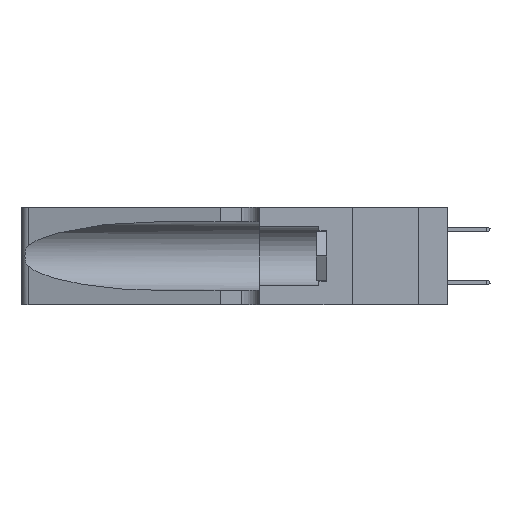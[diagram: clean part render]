
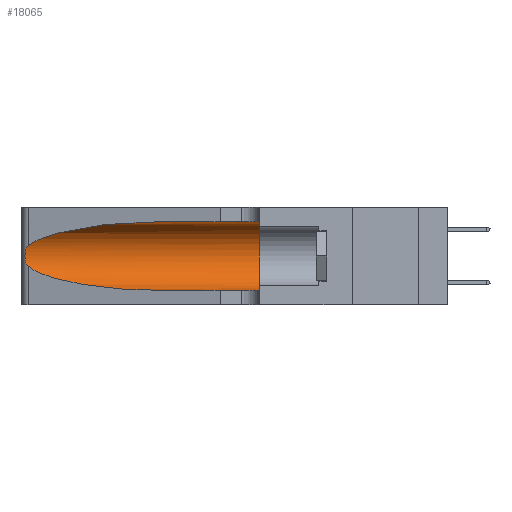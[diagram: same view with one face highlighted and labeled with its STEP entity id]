
A CAD part, left-side view. The second image highlights one B-rep face of the part: STEP entity #18065.
In plain terms, the highlighted cylindrical face has radius 3.308 mm (diameter 6.617 mm), a partial arc.
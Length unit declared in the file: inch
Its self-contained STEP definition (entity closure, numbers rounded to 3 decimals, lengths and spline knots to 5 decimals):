
#172 = CYLINDRICAL_SURFACE ( 'NONE', #28680, 0.13025 ) ;
#810 = CARTESIAN_POINT ( 'NONE',  ( 0.25487, 1.22718, 0.22369 ) ) ;
#1153 = FACE_OUTER_BOUND ( 'NONE', #14754, .T. ) ;
#1333 = CARTESIAN_POINT ( 'NONE',  ( 0.26018, 1.23835, 0.19895 ) ) ;
#2042 = CARTESIAN_POINT ( 'NONE',  ( 0.1305, 0.35, 0.05475 ) ) ;
#2505 = ORIENTED_EDGE ( 'NONE', *, *, #38951, .F. ) ;
#3276 = CIRCLE ( 'NONE', #6187, 0.13025 ) ;
#3531 = CARTESIAN_POINT ( 'NONE',  ( 0.1305, 0.35, 0.185 ) ) ;
#4413 = CARTESIAN_POINT ( 'NONE',  ( 0.26075, 1.23896, 0.178 ) ) ;
#4618 = CARTESIAN_POINT ( 'NONE',  ( 0.1305, 0.72297, 0.05475 ) ) ;
#4902 = ORIENTED_EDGE ( 'NONE', *, *, #29166, .F. ) ;
#6082 = CARTESIAN_POINT ( 'NONE',  ( 0.1305, 1.61858, 0.05475 ) ) ;
#6187 = AXIS2_PLACEMENT_3D ( 'NONE', #3531, #25128, #6649 ) ;
#6359 =( BOUNDED_CURVE ( )  B_SPLINE_CURVE ( 3, ( #38432, #16950, #23096, #4618 ),
 .UNSPECIFIED., .F., .T. ) 
 B_SPLINE_CURVE_WITH_KNOTS ( ( 4, 4 ),
 ( 3.44316, 4.71239 ),
 .UNSPECIFIED. ) 
 CURVE ( )  GEOMETRIC_REPRESENTATION_ITEM ( )  RATIONAL_B_SPLINE_CURVE ( ( 1., 0.87, 0.87, 1. ) ) 
 REPRESENTATION_ITEM ( '' )  );
#6649 = DIRECTION ( 'NONE',  ( 0., 0., 1. ) ) ;
#6908 = CARTESIAN_POINT ( 'NONE',  ( 0.18966, 0.96281, 0.31525 ) ) ;
#7192 = VECTOR ( 'NONE', #23256, 39.37008 ) ;
#7552 = CARTESIAN_POINT ( 'NONE',  ( 0.25856, 1.23593, 0.16098 ) ) ;
#7822 =( BOUNDED_CURVE ( )  B_SPLINE_CURVE ( 3, ( #13120, #6908, #19323, #810 ),
 .UNSPECIFIED., .F., .T. ) 
 B_SPLINE_CURVE_WITH_KNOTS ( ( 4, 4 ),
 ( 1.5708, 2.84003 ),
 .UNSPECIFIED. ) 
 CURVE ( )  GEOMETRIC_REPRESENTATION_ITEM ( )  RATIONAL_B_SPLINE_CURVE ( ( 1., 0.87, 0.87, 1. ) ) 
 REPRESENTATION_ITEM ( '' )  );
#8098 = ORIENTED_EDGE ( 'NONE', *, *, #9304, .T. ) ;
#8523 = ORIENTED_EDGE ( 'NONE', *, *, #10488, .T. ) ;
#9304 = EDGE_CURVE ( 'NONE', #12887, #9495, #32209, .T. ) ;
#9495 = VERTEX_POINT ( 'NONE', #36215 ) ;
#10488 = EDGE_CURVE ( 'NONE', #17435, #12887, #7822, .T. ) ;
#10525 = ORIENTED_EDGE ( 'NONE', *, *, #38538, .T. ) ;
#10658 = CARTESIAN_POINT ( 'NONE',  ( 0.25639, 1.23186, 0.15144 ) ) ;
#10725 = VERTEX_POINT ( 'NONE', #2042 ) ;
#12756 = VERTEX_POINT ( 'NONE', #27336 ) ;
#12887 = VERTEX_POINT ( 'NONE', #21657 ) ;
#13120 = CARTESIAN_POINT ( 'NONE',  ( 0.1305, 0.72297, 0.31525 ) ) ;
#13646 = CARTESIAN_POINT ( 'NONE',  ( 0.25555, 1.22994, 0.2215 ) ) ;
#13783 = CARTESIAN_POINT ( 'NONE',  ( 0.25487, 1.22718, 0.14631 ) ) ;
#14754 = EDGE_LOOP ( 'NONE', ( #8523, #8098, #10525, #37962, #4902, #2505 ) ) ;
#14966 = VERTEX_POINT ( 'NONE', #27499 ) ;
#16735 = CARTESIAN_POINT ( 'NONE',  ( 0.25487, 1.22718, 0.22369 ) ) ;
#16884 = DIRECTION ( 'NONE',  ( 0., 0., -1. ) ) ;
#16950 = CARTESIAN_POINT ( 'NONE',  ( 0.2373, 1.15595, 0.08982 ) ) ;
#17435 = VERTEX_POINT ( 'NONE', #32528 ) ;
#18065 = ADVANCED_FACE ( 'NONE', ( #1153 ), #172, .F. ) ;
#18513 = DIRECTION ( 'NONE',  ( 0., -1., 0. ) ) ;
#19323 = CARTESIAN_POINT ( 'NONE',  ( 0.2373, 1.15595, 0.28018 ) ) ;
#19823 = CARTESIAN_POINT ( 'NONE',  ( 0.25854, 1.2359, 0.20912 ) ) ;
#21657 = CARTESIAN_POINT ( 'NONE',  ( 0.25487, 1.22718, 0.22369 ) ) ;
#22182 = VECTOR ( 'NONE', #18513, 39.37008 ) ;
#22871 = CARTESIAN_POINT ( 'NONE',  ( 0.26075, 1.23896, 0.19203 ) ) ;
#23096 = CARTESIAN_POINT ( 'NONE',  ( 0.18966, 0.96281, 0.05475 ) ) ;
#23256 = DIRECTION ( 'NONE',  ( 0., -1., 0. ) ) ;
#25128 = DIRECTION ( 'NONE',  ( 0., 1., 0. ) ) ;
#25350 = LINE ( 'NONE', #38593, #7192 ) ;
#25990 = CARTESIAN_POINT ( 'NONE',  ( 0.26017, 1.23833, 0.17102 ) ) ;
#27336 = CARTESIAN_POINT ( 'NONE',  ( 0.1305, 0.35, 0.31525 ) ) ;
#27499 = CARTESIAN_POINT ( 'NONE',  ( 0.1305, 0.72297, 0.05475 ) ) ;
#28680 = AXIS2_PLACEMENT_3D ( 'NONE', #32208, #29233, #16884 ) ;
#29087 = CARTESIAN_POINT ( 'NONE',  ( 0.25789, 1.23486, 0.15765 ) ) ;
#29166 = EDGE_CURVE ( 'NONE', #12756, #10725, #3276, .T. ) ;
#29233 = DIRECTION ( 'NONE',  ( 0., -1., 0. ) ) ;
#30190 = EDGE_CURVE ( 'NONE', #14966, #10725, #31337, .T. ) ;
#31337 = LINE ( 'NONE', #6082, #22182 ) ;
#32057 = CARTESIAN_POINT ( 'NONE',  ( 0.25639, 1.23184, 0.21858 ) ) ;
#32193 = CARTESIAN_POINT ( 'NONE',  ( 0.25555, 1.22993, 0.14849 ) ) ;
#32208 = CARTESIAN_POINT ( 'NONE',  ( 0.1305, 1.61858, 0.185 ) ) ;
#32209 = B_SPLINE_CURVE_WITH_KNOTS ( 'NONE', 3,
 ( #16735, #13646, #32057, #38234, #19823, #1333, #22871, #4413, #25990, #7552, #29087, #10658, #32193, #13783 ),
 .UNSPECIFIED., .F., .F.,
 ( 4, 2, 2, 2, 2, 2, 4 ),
 ( 0., 0.00027, 0.00053, 0.00107, 0.0016, 0.00187, 0.00214 ),
 .UNSPECIFIED. ) ;
#32528 = CARTESIAN_POINT ( 'NONE',  ( 0.1305, 0.72297, 0.31525 ) ) ;
#36215 = CARTESIAN_POINT ( 'NONE',  ( 0.25487, 1.22718, 0.14631 ) ) ;
#37962 = ORIENTED_EDGE ( 'NONE', *, *, #30190, .T. ) ;
#38234 = CARTESIAN_POINT ( 'NONE',  ( 0.25787, 1.23484, 0.2124 ) ) ;
#38432 = CARTESIAN_POINT ( 'NONE',  ( 0.25487, 1.22718, 0.14631 ) ) ;
#38538 = EDGE_CURVE ( 'NONE', #9495, #14966, #6359, .T. ) ;
#38593 = CARTESIAN_POINT ( 'NONE',  ( 0.1305, 1.61858, 0.31525 ) ) ;
#38951 = EDGE_CURVE ( 'NONE', #17435, #12756, #25350, .T. ) ;
